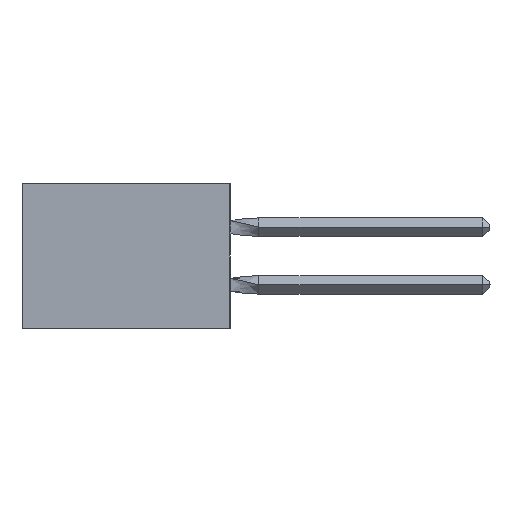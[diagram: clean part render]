
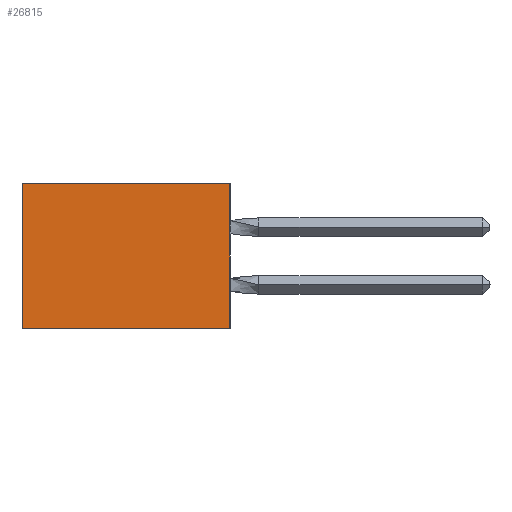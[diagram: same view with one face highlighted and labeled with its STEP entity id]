
A CAD part, left-side view. The second image highlights one B-rep face of the part: STEP entity #26815.
In plain terms, the highlighted planar face has unit normal (-1, 0, 0).
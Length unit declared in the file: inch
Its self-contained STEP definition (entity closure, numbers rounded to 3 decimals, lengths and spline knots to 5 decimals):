
#637 = VECTOR ( 'NONE', #4509, 39.37008 ) ;
#640 = DIRECTION ( 'NONE',  ( 0., 0., -1. ) ) ;
#1009 = VECTOR ( 'NONE', #18026, 39.37008 ) ;
#1155 = CARTESIAN_POINT ( 'NONE',  ( 0.305, 0.72, -0.5 ) ) ;
#2297 = EDGE_CURVE ( 'NONE', #30533, #25275, #18159, .T. ) ;
#2309 = DIRECTION ( 'NONE',  ( 0., 1., 0. ) ) ;
#3996 = CARTESIAN_POINT ( 'NONE',  ( 0.305, 0., -0.5 ) ) ;
#4509 = DIRECTION ( 'NONE',  ( 0., 0., -1. ) ) ;
#5095 = LINE ( 'NONE', #27249, #42869 ) ;
#5437 = EDGE_CURVE ( 'NONE', #30533, #25220, #5095, .T. ) ;
#7542 = FACE_OUTER_BOUND ( 'NONE', #10415, .T. ) ;
#8785 = EDGE_CURVE ( 'NONE', #25275, #34074, #24274, .T. ) ;
#10415 = EDGE_LOOP ( 'NONE', ( #17183, #21016, #17576, #28224 ) ) ;
#15224 = CARTESIAN_POINT ( 'NONE',  ( 0.305, 0., -0.5 ) ) ;
#17183 = ORIENTED_EDGE ( 'NONE', *, *, #31282, .T. ) ;
#17576 = ORIENTED_EDGE ( 'NONE', *, *, #2297, .F. ) ;
#18026 = DIRECTION ( 'NONE',  ( 0., 1., 0. ) ) ;
#18159 = LINE ( 'NONE', #22232, #36523 ) ;
#21016 = ORIENTED_EDGE ( 'NONE', *, *, #8785, .F. ) ;
#22232 = CARTESIAN_POINT ( 'NONE',  ( 0.305, 0., -0.5 ) ) ;
#24274 = LINE ( 'NONE', #36056, #1009 ) ;
#25220 = VERTEX_POINT ( 'NONE', #39655 ) ;
#25253 = PLANE ( 'NONE',  #29869 ) ;
#25275 = VERTEX_POINT ( 'NONE', #15224 ) ;
#26072 = DIRECTION ( 'NONE',  ( 0., 0., -1. ) ) ;
#26815 = ADVANCED_FACE ( 'NONE', ( #7542 ), #25253, .F. ) ;
#27249 = CARTESIAN_POINT ( 'NONE',  ( 0.305, 0., 0. ) ) ;
#28224 = ORIENTED_EDGE ( 'NONE', *, *, #5437, .T. ) ;
#29869 = AXIS2_PLACEMENT_3D ( 'NONE', #3996, #32426, #640 ) ;
#30533 = VERTEX_POINT ( 'NONE', #39547 ) ;
#31282 = EDGE_CURVE ( 'NONE', #25220, #34074, #36215, .T. ) ;
#32426 = DIRECTION ( 'NONE',  ( 1., 0., 0. ) ) ;
#34074 = VERTEX_POINT ( 'NONE', #43539 ) ;
#36056 = CARTESIAN_POINT ( 'NONE',  ( 0.305, 0., -0.5 ) ) ;
#36215 = LINE ( 'NONE', #1155, #637 ) ;
#36523 = VECTOR ( 'NONE', #26072, 39.37008 ) ;
#39547 = CARTESIAN_POINT ( 'NONE',  ( 0.305, 0., 0. ) ) ;
#39655 = CARTESIAN_POINT ( 'NONE',  ( 0.305, 0.72, 0. ) ) ;
#42869 = VECTOR ( 'NONE', #2309, 39.37008 ) ;
#43539 = CARTESIAN_POINT ( 'NONE',  ( 0.305, 0.72, -0.5 ) ) ;
